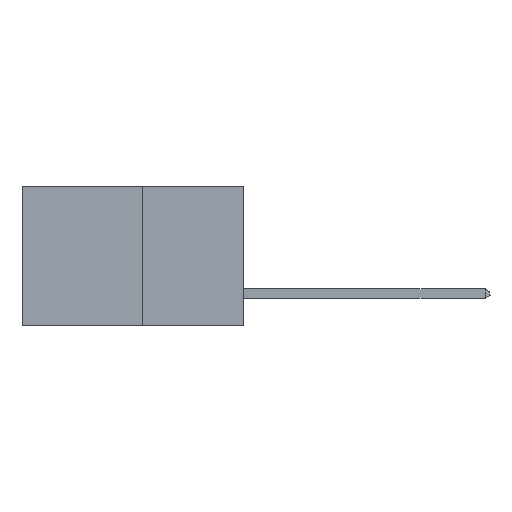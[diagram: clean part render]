
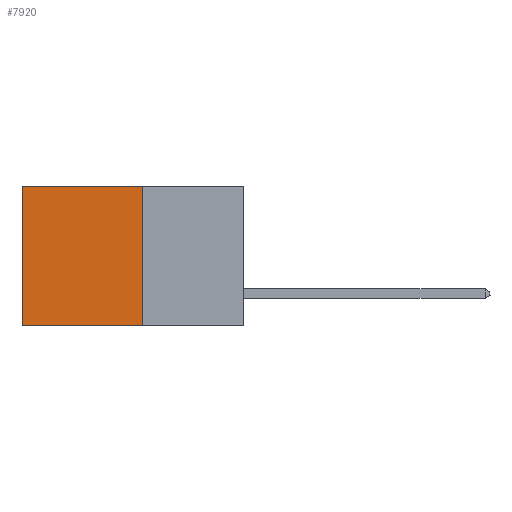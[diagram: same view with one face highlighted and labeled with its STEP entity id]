
A CAD part, left-side view. The second image highlights one B-rep face of the part: STEP entity #7920.
In plain terms, the highlighted planar face has unit normal (-1, 0, 0).
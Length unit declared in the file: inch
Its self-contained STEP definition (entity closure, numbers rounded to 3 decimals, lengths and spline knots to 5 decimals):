
#421 = VECTOR ( 'NONE', #19979, 39.37008 ) ;
#1408 = ORIENTED_EDGE ( 'NONE', *, *, #19512, .T. ) ;
#2300 = VECTOR ( 'NONE', #27049, 39.37008 ) ;
#2329 = VERTEX_POINT ( 'NONE', #11730 ) ;
#2656 = AXIS2_PLACEMENT_3D ( 'NONE', #22323, #24307, #12119 ) ;
#5113 = CARTESIAN_POINT ( 'NONE',  ( 0.277, 0.59, -0.37 ) ) ;
#6035 = CARTESIAN_POINT ( 'NONE',  ( 0.277, 0.27, 0. ) ) ;
#6394 = CARTESIAN_POINT ( 'NONE',  ( 0.277, 0.27, -0.37 ) ) ;
#6857 = EDGE_LOOP ( 'NONE', ( #1408, #15184, #21973, #10486 ) ) ;
#6893 = DIRECTION ( 'NONE',  ( 0., 0., -1. ) ) ;
#7449 = VECTOR ( 'NONE', #20833, 39.37008 ) ;
#7476 = LINE ( 'NONE', #6394, #2300 ) ;
#7688 = CARTESIAN_POINT ( 'NONE',  ( 0.277, 0.59, 0. ) ) ;
#7920 = ADVANCED_FACE ( 'NONE', ( #11307 ), #18268, .F. ) ;
#9709 = VERTEX_POINT ( 'NONE', #21430 ) ;
#10034 = VERTEX_POINT ( 'NONE', #16893 ) ;
#10486 = ORIENTED_EDGE ( 'NONE', *, *, #16786, .T. ) ;
#11307 = FACE_OUTER_BOUND ( 'NONE', #6857, .T. ) ;
#11730 = CARTESIAN_POINT ( 'NONE',  ( 0.277, 0.27, 0. ) ) ;
#12119 = DIRECTION ( 'NONE',  ( 0., 0., -1. ) ) ;
#14593 = LINE ( 'NONE', #19586, #20057 ) ;
#15184 = ORIENTED_EDGE ( 'NONE', *, *, #23572, .F. ) ;
#16786 = EDGE_CURVE ( 'NONE', #2329, #20238, #19352, .T. ) ;
#16893 = CARTESIAN_POINT ( 'NONE',  ( 0.277, 0.27, -0.37 ) ) ;
#16980 = LINE ( 'NONE', #5113, #421 ) ;
#18268 = PLANE ( 'NONE',  #2656 ) ;
#19352 = LINE ( 'NONE', #6035, #7449 ) ;
#19512 = EDGE_CURVE ( 'NONE', #20238, #9709, #16980, .T. ) ;
#19586 = CARTESIAN_POINT ( 'NONE',  ( 0.277, 0.27, -0.37 ) ) ;
#19979 = DIRECTION ( 'NONE',  ( 0., 0., -1. ) ) ;
#20057 = VECTOR ( 'NONE', #6893, 39.37008 ) ;
#20238 = VERTEX_POINT ( 'NONE', #7688 ) ;
#20833 = DIRECTION ( 'NONE',  ( 0., 1., 0. ) ) ;
#21430 = CARTESIAN_POINT ( 'NONE',  ( 0.277, 0.59, -0.37 ) ) ;
#21973 = ORIENTED_EDGE ( 'NONE', *, *, #23707, .F. ) ;
#22323 = CARTESIAN_POINT ( 'NONE',  ( 0.277, 0.27, -0.37 ) ) ;
#23572 = EDGE_CURVE ( 'NONE', #10034, #9709, #7476, .T. ) ;
#23707 = EDGE_CURVE ( 'NONE', #2329, #10034, #14593, .T. ) ;
#24307 = DIRECTION ( 'NONE',  ( 1., 0., 0. ) ) ;
#27049 = DIRECTION ( 'NONE',  ( 0., 1., 0. ) ) ;
